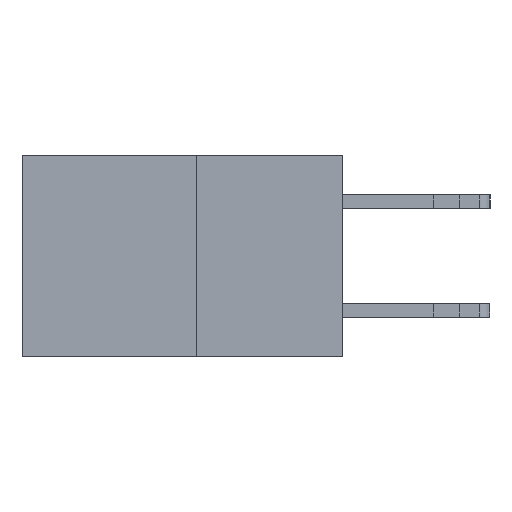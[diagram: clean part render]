
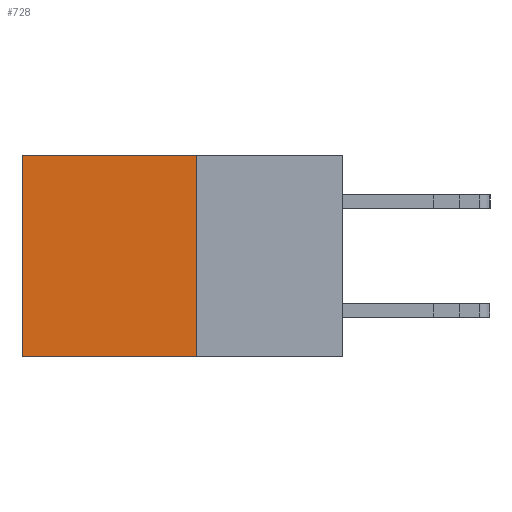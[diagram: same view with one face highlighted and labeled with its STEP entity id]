
A CAD part, left-side view. The second image highlights one B-rep face of the part: STEP entity #728.
In plain terms, the highlighted planar face has unit normal (-1, 0, 0).
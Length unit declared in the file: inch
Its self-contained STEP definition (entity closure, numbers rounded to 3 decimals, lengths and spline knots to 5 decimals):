
#498 = EDGE_CURVE ( 'NONE', #1455, #12671, #5003, .T. ) ;
#624 = ORIENTED_EDGE ( 'NONE', *, *, #14578, .F. ) ;
#728 = ADVANCED_FACE ( 'NONE', ( #4820 ), #1623, .F. ) ;
#935 = DIRECTION ( 'NONE',  ( 0., 1., 0. ) ) ;
#1455 = VERTEX_POINT ( 'NONE', #7398 ) ;
#1623 = PLANE ( 'NONE',  #8938 ) ;
#1633 = LINE ( 'NONE', #15759, #14145 ) ;
#1862 = VECTOR ( 'NONE', #13516, 39.37008 ) ;
#1998 = DIRECTION ( 'NONE',  ( 0., 0., -1. ) ) ;
#2304 = CARTESIAN_POINT ( 'NONE',  ( 0.277, 0.27, -0.37 ) ) ;
#3749 = CARTESIAN_POINT ( 'NONE',  ( 0.277, 0.59, -0.37 ) ) ;
#4612 = CARTESIAN_POINT ( 'NONE',  ( 0.277, 0.27, -0.37 ) ) ;
#4820 = FACE_OUTER_BOUND ( 'NONE', #14587, .T. ) ;
#5003 = LINE ( 'NONE', #7992, #14486 ) ;
#5218 = LINE ( 'NONE', #13535, #1862 ) ;
#6202 = ORIENTED_EDGE ( 'NONE', *, *, #498, .T. ) ;
#6398 = EDGE_CURVE ( 'NONE', #13202, #1455, #5218, .T. ) ;
#6643 = EDGE_CURVE ( 'NONE', #13202, #10302, #1633, .T. ) ;
#6837 = ORIENTED_EDGE ( 'NONE', *, *, #6643, .F. ) ;
#7288 = CARTESIAN_POINT ( 'NONE',  ( 0.277, 0.27, -0.37 ) ) ;
#7292 = LINE ( 'NONE', #7288, #13894 ) ;
#7398 = CARTESIAN_POINT ( 'NONE',  ( 0.277, 0.59, 0. ) ) ;
#7812 = ORIENTED_EDGE ( 'NONE', *, *, #6398, .T. ) ;
#7992 = CARTESIAN_POINT ( 'NONE',  ( 0.277, 0.59, -0.37 ) ) ;
#8316 = CARTESIAN_POINT ( 'NONE',  ( 0.277, 0.27, 0. ) ) ;
#8938 = AXIS2_PLACEMENT_3D ( 'NONE', #2304, #9102, #1998 ) ;
#9102 = DIRECTION ( 'NONE',  ( 1., 0., 0. ) ) ;
#10302 = VERTEX_POINT ( 'NONE', #4612 ) ;
#11806 = DIRECTION ( 'NONE',  ( 0., 0., -1. ) ) ;
#12671 = VERTEX_POINT ( 'NONE', #3749 ) ;
#13202 = VERTEX_POINT ( 'NONE', #8316 ) ;
#13516 = DIRECTION ( 'NONE',  ( 0., 1., 0. ) ) ;
#13535 = CARTESIAN_POINT ( 'NONE',  ( 0.277, 0.27, 0. ) ) ;
#13894 = VECTOR ( 'NONE', #935, 39.37008 ) ;
#14145 = VECTOR ( 'NONE', #15632, 39.37008 ) ;
#14486 = VECTOR ( 'NONE', #11806, 39.37008 ) ;
#14578 = EDGE_CURVE ( 'NONE', #10302, #12671, #7292, .T. ) ;
#14587 = EDGE_LOOP ( 'NONE', ( #6202, #624, #6837, #7812 ) ) ;
#15632 = DIRECTION ( 'NONE',  ( 0., 0., -1. ) ) ;
#15759 = CARTESIAN_POINT ( 'NONE',  ( 0.277, 0.27, -0.37 ) ) ;
